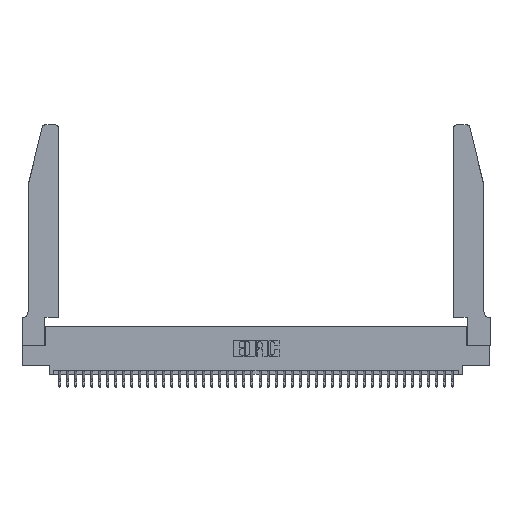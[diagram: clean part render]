
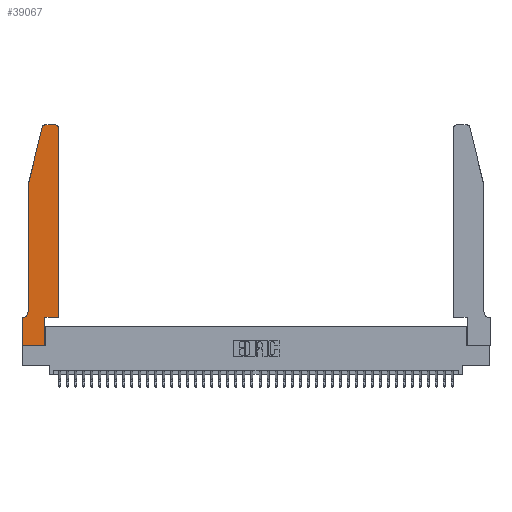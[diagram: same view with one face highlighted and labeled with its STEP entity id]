
A CAD part, top view. The second image highlights one B-rep face of the part: STEP entity #39067.
In plain terms, the highlighted planar face has unit normal (0, 0, 1).
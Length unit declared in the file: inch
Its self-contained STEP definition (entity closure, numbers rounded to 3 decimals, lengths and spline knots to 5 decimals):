
#125 = ORIENTED_EDGE ( 'NONE', *, *, #23927, .T. ) ;
#255 = VECTOR ( 'NONE', #42674, 39.37008 ) ;
#423 = DIRECTION ( 'NONE',  ( 0., 0., 1. ) ) ;
#686 = VECTOR ( 'NONE', #28359, 39.37008 ) ;
#760 = CARTESIAN_POINT ( 'NONE',  ( 0.4505, 0.35, 0.37 ) ) ;
#2079 = EDGE_CURVE ( 'NONE', #20664, #5574, #43032, .T. ) ;
#2657 = VERTEX_POINT ( 'NONE', #33055 ) ;
#2926 = AXIS2_PLACEMENT_3D ( 'NONE', #37251, #40620, #10669 ) ;
#3030 = EDGE_CURVE ( 'NONE', #5574, #14819, #30868, .T. ) ;
#4266 = FACE_OUTER_BOUND ( 'NONE', #36482, .T. ) ;
#4512 = DIRECTION ( 'NONE',  ( -1., 0., 0. ) ) ;
#4955 = CARTESIAN_POINT ( 'NONE',  ( 0.4505, 0.35, 0.37 ) ) ;
#5112 = DIRECTION ( 'NONE',  ( -1., 0., 0. ) ) ;
#5574 = VERTEX_POINT ( 'NONE', #22776 ) ;
#5946 = VERTEX_POINT ( 'NONE', #14945 ) ;
#5995 = LINE ( 'NONE', #32300, #255 ) ;
#7001 = DIRECTION ( 'NONE',  ( 0., 0., -1. ) ) ;
#7735 = AXIS2_PLACEMENT_3D ( 'NONE', #23715, #7001, #13740 ) ;
#8295 = ORIENTED_EDGE ( 'NONE', *, *, #2079, .T. ) ;
#8875 = CARTESIAN_POINT ( 'NONE',  ( 0.2605, 2.75, 0.37 ) ) ;
#9303 = LINE ( 'NONE', #10275, #25606 ) ;
#10275 = CARTESIAN_POINT ( 'NONE',  ( 0.4505, 0.35, 0.37 ) ) ;
#10669 = DIRECTION ( 'NONE',  ( 1., 0., 0. ) ) ;
#10764 = DIRECTION ( 'NONE',  ( 0., -1., 0. ) ) ;
#10903 = CARTESIAN_POINT ( 'NONE',  ( 0.4205, 2.72, 0.37 ) ) ;
#11079 = VERTEX_POINT ( 'NONE', #30002 ) ;
#11462 = CARTESIAN_POINT ( 'NONE',  ( 0.0055, 0.35, 0.37 ) ) ;
#11710 = VERTEX_POINT ( 'NONE', #11462 ) ;
#13100 = VECTOR ( 'NONE', #26439, 39.37008 ) ;
#13740 = DIRECTION ( 'NONE',  ( -1., 0., 0. ) ) ;
#14046 = CARTESIAN_POINT ( 'NONE',  ( 0., 0.35, 0.37 ) ) ;
#14819 = VERTEX_POINT ( 'NONE', #23572 ) ;
#14945 = CARTESIAN_POINT ( 'NONE',  ( 0., 0., 0.37 ) ) ;
#15312 = VECTOR ( 'NONE', #18246, 39.37008 ) ;
#15902 = CARTESIAN_POINT ( 'NONE',  ( 0.4505, 2.72, 0.37 ) ) ;
#16630 = VERTEX_POINT ( 'NONE', #15902 ) ;
#17190 = EDGE_CURVE ( 'NONE', #35638, #5946, #42871, .T. ) ;
#17291 = DIRECTION ( 'NONE',  ( 0., 0., 1. ) ) ;
#17830 = CARTESIAN_POINT ( 'NONE',  ( 0., 0.35, 0.37 ) ) ;
#18246 = DIRECTION ( 'NONE',  ( 0., 1., 0. ) ) ;
#18322 = ORIENTED_EDGE ( 'NONE', *, *, #3030, .T. ) ;
#19379 = CARTESIAN_POINT ( 'NONE',  ( 0., 0., 0.37 ) ) ;
#20059 = CARTESIAN_POINT ( 'NONE',  ( 0.4205, 2.75, 0.37 ) ) ;
#20504 = DIRECTION ( 'NONE',  ( 1., 0., 0. ) ) ;
#20664 = VERTEX_POINT ( 'NONE', #20059 ) ;
#21236 = ORIENTED_EDGE ( 'NONE', *, *, #28640, .T. ) ;
#21543 = ORIENTED_EDGE ( 'NONE', *, *, #34317, .T. ) ;
#21590 = ORIENTED_EDGE ( 'NONE', *, *, #34884, .T. ) ;
#22628 = EDGE_CURVE ( 'NONE', #14819, #37873, #5995, .T. ) ;
#22776 = CARTESIAN_POINT ( 'NONE',  ( 0.284, 2.75, 0.37 ) ) ;
#23100 = VERTEX_POINT ( 'NONE', #760 ) ;
#23337 = CARTESIAN_POINT ( 'NONE',  ( 0., 0., 0.37 ) ) ;
#23572 = CARTESIAN_POINT ( 'NONE',  ( 0.25487, 2.72718, 0.37 ) ) ;
#23715 = CARTESIAN_POINT ( 'NONE',  ( 0.0055, 0.42, 0.37 ) ) ;
#23927 = EDGE_CURVE ( 'NONE', #27229, #11079, #39348, .T. ) ;
#24049 = LINE ( 'NONE', #37501, #37594 ) ;
#25606 = VECTOR ( 'NONE', #36618, 39.37008 ) ;
#25773 = AXIS2_PLACEMENT_3D ( 'NONE', #14046, #17291, #20504 ) ;
#25893 = CIRCLE ( 'NONE', #43206, 0.03 ) ;
#26024 = EDGE_CURVE ( 'NONE', #2657, #11710, #38104, .T. ) ;
#26439 = DIRECTION ( 'NONE',  ( 1., 0., 0. ) ) ;
#26838 = ORIENTED_EDGE ( 'NONE', *, *, #26024, .T. ) ;
#26981 = CARTESIAN_POINT ( 'NONE',  ( 0.2865, 0., 0.37 ) ) ;
#27042 = EDGE_CURVE ( 'NONE', #11710, #35638, #35941, .T. ) ;
#27215 = ORIENTED_EDGE ( 'NONE', *, *, #17190, .T. ) ;
#27229 = VERTEX_POINT ( 'NONE', #26981 ) ;
#27671 = VECTOR ( 'NONE', #42834, 39.37008 ) ;
#28359 = DIRECTION ( 'NONE',  ( 0., 1., 0. ) ) ;
#28640 = EDGE_CURVE ( 'NONE', #16630, #20664, #25893, .T. ) ;
#30002 = CARTESIAN_POINT ( 'NONE',  ( 0.2865, 0.35, 0.37 ) ) ;
#30336 = LINE ( 'NONE', #19379, #13100 ) ;
#30868 = CIRCLE ( 'NONE', #2926, 0.03 ) ;
#32300 = CARTESIAN_POINT ( 'NONE',  ( 0.0755, 2., 0.37 ) ) ;
#32352 = ORIENTED_EDGE ( 'NONE', *, *, #38094, .T. ) ;
#33055 = CARTESIAN_POINT ( 'NONE',  ( 0.0755, 0.42, 0.37 ) ) ;
#33168 = LINE ( 'NONE', #4955, #686 ) ;
#33583 = ORIENTED_EDGE ( 'NONE', *, *, #40246, .T. ) ;
#34040 = CARTESIAN_POINT ( 'NONE',  ( 0.0755, 0.35, 0.37 ) ) ;
#34102 = VECTOR ( 'NONE', #5112, 39.37008 ) ;
#34112 = PLANE ( 'NONE',  #25773 ) ;
#34317 = EDGE_CURVE ( 'NONE', #37873, #2657, #24049, .T. ) ;
#34884 = EDGE_CURVE ( 'NONE', #11079, #23100, #9303, .T. ) ;
#35638 = VERTEX_POINT ( 'NONE', #17830 ) ;
#35941 = LINE ( 'NONE', #34040, #38530 ) ;
#36482 = EDGE_LOOP ( 'NONE', ( #8295, #18322, #37186, #21543, #26838, #37581, #27215, #33583, #125, #21590, #32352, #21236 ) ) ;
#36618 = DIRECTION ( 'NONE',  ( 1., 0., 0. ) ) ;
#37186 = ORIENTED_EDGE ( 'NONE', *, *, #22628, .T. ) ;
#37251 = CARTESIAN_POINT ( 'NONE',  ( 0.284, 2.72, 0.37 ) ) ;
#37501 = CARTESIAN_POINT ( 'NONE',  ( 0.0755, 2., 0.37 ) ) ;
#37581 = ORIENTED_EDGE ( 'NONE', *, *, #27042, .T. ) ;
#37594 = VECTOR ( 'NONE', #10764, 39.37008 ) ;
#37873 = VERTEX_POINT ( 'NONE', #40585 ) ;
#38094 = EDGE_CURVE ( 'NONE', #23100, #16630, #33168, .T. ) ;
#38104 = CIRCLE ( 'NONE', #7735, 0.07 ) ;
#38530 = VECTOR ( 'NONE', #4512, 39.37008 ) ;
#39067 = ADVANCED_FACE ( 'NONE', ( #4266 ), #34112, .T. ) ;
#39348 = LINE ( 'NONE', #41351, #15312 ) ;
#40246 = EDGE_CURVE ( 'NONE', #5946, #27229, #30336, .T. ) ;
#40585 = CARTESIAN_POINT ( 'NONE',  ( 0.0755, 2., 0.37 ) ) ;
#40620 = DIRECTION ( 'NONE',  ( 0., 0., 1. ) ) ;
#40966 = DIRECTION ( 'NONE',  ( 1., 0., 0. ) ) ;
#41351 = CARTESIAN_POINT ( 'NONE',  ( 0.2865, 0.35, 0.37 ) ) ;
#42674 = DIRECTION ( 'NONE',  ( -0.239, -0.971, 0. ) ) ;
#42834 = DIRECTION ( 'NONE',  ( 0., -1., 0. ) ) ;
#42871 = LINE ( 'NONE', #23337, #27671 ) ;
#43032 = LINE ( 'NONE', #8875, #34102 ) ;
#43206 = AXIS2_PLACEMENT_3D ( 'NONE', #10903, #423, #40966 ) ;
